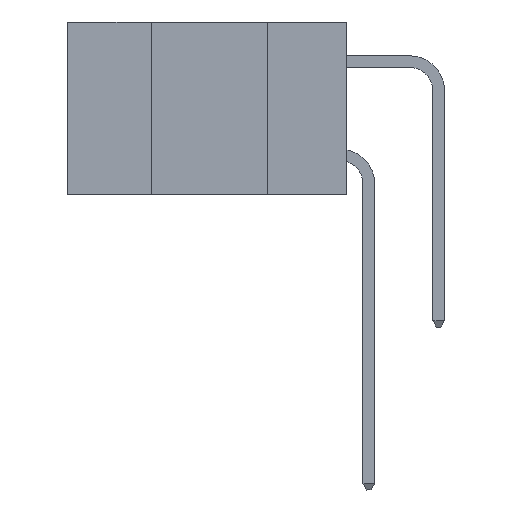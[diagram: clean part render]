
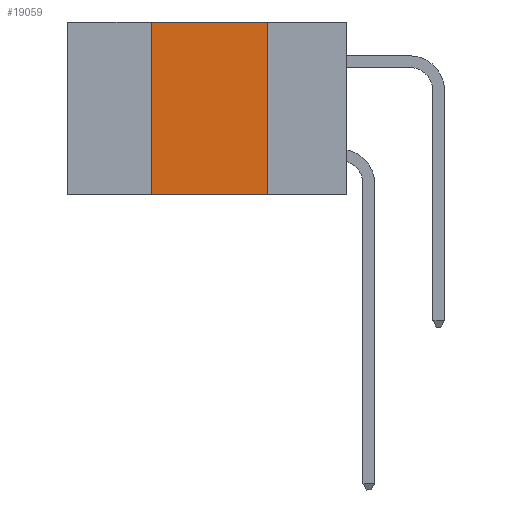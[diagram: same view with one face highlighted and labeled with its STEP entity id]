
A CAD part, left-side view. The second image highlights one B-rep face of the part: STEP entity #19059.
In plain terms, the highlighted planar face has unit normal (-1, 0, 0).
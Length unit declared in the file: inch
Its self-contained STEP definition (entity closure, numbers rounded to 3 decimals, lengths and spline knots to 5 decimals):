
#792 = EDGE_LOOP ( 'NONE', ( #17534, #8404, #7468, #18478 ) ) ;
#1348 = AXIS2_PLACEMENT_3D ( 'NONE', #19853, #8178, #21856 ) ;
#3068 = CARTESIAN_POINT ( 'NONE',  ( 0., 0.6, 0. ) ) ;
#4136 = VECTOR ( 'NONE', #24890, 39.37008 ) ;
#4450 = LINE ( 'NONE', #5345, #20319 ) ;
#4600 = VECTOR ( 'NONE', #14103, 39.37008 ) ;
#5345 = CARTESIAN_POINT ( 'NONE',  ( 0., 0.42, 0. ) ) ;
#5487 = CARTESIAN_POINT ( 'NONE',  ( 0., 0.17, -0.37 ) ) ;
#6165 = PLANE ( 'NONE',  #1348 ) ;
#6299 = CARTESIAN_POINT ( 'NONE',  ( 0., 0.17, 0. ) ) ;
#7468 = ORIENTED_EDGE ( 'NONE', *, *, #10560, .F. ) ;
#7878 = VERTEX_POINT ( 'NONE', #13052 ) ;
#8178 = DIRECTION ( 'NONE',  ( 1., 0., 0. ) ) ;
#8244 = LINE ( 'NONE', #3068, #18010 ) ;
#8404 = ORIENTED_EDGE ( 'NONE', *, *, #20896, .F. ) ;
#9276 = EDGE_CURVE ( 'NONE', #16091, #25360, #15166, .T. ) ;
#10560 = EDGE_CURVE ( 'NONE', #16091, #7878, #4450, .T. ) ;
#11866 = EDGE_CURVE ( 'NONE', #22229, #25360, #25393, .T. ) ;
#13052 = CARTESIAN_POINT ( 'NONE',  ( 0., 0.42, 0. ) ) ;
#13256 = DIRECTION ( 'NONE',  ( 0., 0., 1. ) ) ;
#14103 = DIRECTION ( 'NONE',  ( 0., 0., -1. ) ) ;
#14939 = DIRECTION ( 'NONE',  ( 0., -1., 0. ) ) ;
#15166 = LINE ( 'NONE', #22993, #4136 ) ;
#16091 = VERTEX_POINT ( 'NONE', #19924 ) ;
#17534 = ORIENTED_EDGE ( 'NONE', *, *, #11866, .F. ) ;
#18010 = VECTOR ( 'NONE', #14939, 39.37008 ) ;
#18478 = ORIENTED_EDGE ( 'NONE', *, *, #9276, .T. ) ;
#18606 = FACE_OUTER_BOUND ( 'NONE', #792, .T. ) ;
#19059 = ADVANCED_FACE ( 'NONE', ( #18606 ), #6165, .F. ) ;
#19853 = CARTESIAN_POINT ( 'NONE',  ( 0., 0.6, 0. ) ) ;
#19924 = CARTESIAN_POINT ( 'NONE',  ( 0., 0.42, -0.37 ) ) ;
#20319 = VECTOR ( 'NONE', #13256, 39.37008 ) ;
#20896 = EDGE_CURVE ( 'NONE', #7878, #22229, #8244, .T. ) ;
#21856 = DIRECTION ( 'NONE',  ( 0., 0., -1. ) ) ;
#22229 = VERTEX_POINT ( 'NONE', #25017 ) ;
#22993 = CARTESIAN_POINT ( 'NONE',  ( 0., 0.6, -0.37 ) ) ;
#24890 = DIRECTION ( 'NONE',  ( 0., -1., 0. ) ) ;
#25017 = CARTESIAN_POINT ( 'NONE',  ( 0., 0.17, 0. ) ) ;
#25360 = VERTEX_POINT ( 'NONE', #5487 ) ;
#25393 = LINE ( 'NONE', #6299, #4600 ) ;
